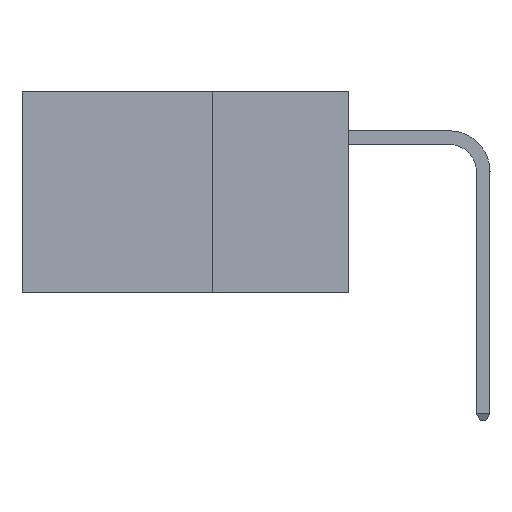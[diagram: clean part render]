
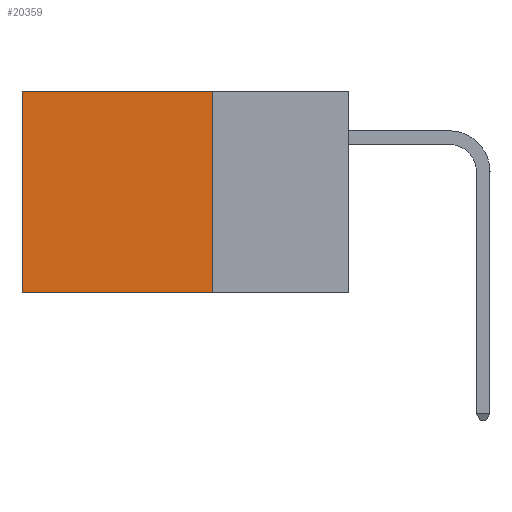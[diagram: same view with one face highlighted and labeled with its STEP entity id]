
A CAD part, left-side view. The second image highlights one B-rep face of the part: STEP entity #20359.
In plain terms, the highlighted planar face has unit normal (-1, 0, 0).
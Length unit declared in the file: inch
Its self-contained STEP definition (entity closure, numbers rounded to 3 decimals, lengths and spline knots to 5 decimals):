
#674 = VECTOR ( 'NONE', #28462, 39.37008 ) ;
#1531 = LINE ( 'NONE', #1655, #30522 ) ;
#1655 = CARTESIAN_POINT ( 'NONE',  ( 0.2875, 0.25, 0. ) ) ;
#2273 = DIRECTION ( 'NONE',  ( 0., 0., -1. ) ) ;
#3251 = CARTESIAN_POINT ( 'NONE',  ( 0.2875, 0.25, 0. ) ) ;
#4629 = VECTOR ( 'NONE', #25604, 39.37008 ) ;
#7291 = CARTESIAN_POINT ( 'NONE',  ( 0.2875, 0.25, -0.37 ) ) ;
#10611 = DIRECTION ( 'NONE',  ( 0., 1., 0. ) ) ;
#13455 = ORIENTED_EDGE ( 'NONE', *, *, #17270, .F. ) ;
#13987 = CARTESIAN_POINT ( 'NONE',  ( 0.2875, 0.25, -0.37 ) ) ;
#14924 = EDGE_CURVE ( 'NONE', #35983, #22302, #40123, .T. ) ;
#17270 = EDGE_CURVE ( 'NONE', #39607, #22302, #33731, .T. ) ;
#20359 = ADVANCED_FACE ( 'NONE', ( #41678 ), #40461, .F. ) ;
#22302 = VERTEX_POINT ( 'NONE', #36158 ) ;
#24394 = LINE ( 'NONE', #47756, #674 ) ;
#24557 = EDGE_LOOP ( 'NONE', ( #26845, #13455, #37991, #33889 ) ) ;
#25604 = DIRECTION ( 'NONE',  ( 0., 0., -1. ) ) ;
#26241 = EDGE_CURVE ( 'NONE', #45452, #35983, #1531, .T. ) ;
#26606 = VECTOR ( 'NONE', #10611, 39.37008 ) ;
#26845 = ORIENTED_EDGE ( 'NONE', *, *, #14924, .T. ) ;
#28206 = EDGE_CURVE ( 'NONE', #45452, #39607, #24394, .T. ) ;
#28462 = DIRECTION ( 'NONE',  ( 0., 0., -1. ) ) ;
#29075 = DIRECTION ( 'NONE',  ( 1., 0., 0. ) ) ;
#29636 = CARTESIAN_POINT ( 'NONE',  ( 0.2875, 0.6, 0. ) ) ;
#30522 = VECTOR ( 'NONE', #31423, 39.37008 ) ;
#31423 = DIRECTION ( 'NONE',  ( 0., 1., 0. ) ) ;
#33731 = LINE ( 'NONE', #7291, #26606 ) ;
#33889 = ORIENTED_EDGE ( 'NONE', *, *, #26241, .T. ) ;
#35983 = VERTEX_POINT ( 'NONE', #29636 ) ;
#36158 = CARTESIAN_POINT ( 'NONE',  ( 0.2875, 0.6, -0.37 ) ) ;
#37991 = ORIENTED_EDGE ( 'NONE', *, *, #28206, .F. ) ;
#39607 = VERTEX_POINT ( 'NONE', #13987 ) ;
#39979 = CARTESIAN_POINT ( 'NONE',  ( 0.2875, 0.25, 0. ) ) ;
#40123 = LINE ( 'NONE', #40622, #4629 ) ;
#40461 = PLANE ( 'NONE',  #46974 ) ;
#40622 = CARTESIAN_POINT ( 'NONE',  ( 0.2875, 0.6, 0. ) ) ;
#41678 = FACE_OUTER_BOUND ( 'NONE', #24557, .T. ) ;
#45452 = VERTEX_POINT ( 'NONE', #3251 ) ;
#46974 = AXIS2_PLACEMENT_3D ( 'NONE', #39979, #29075, #2273 ) ;
#47756 = CARTESIAN_POINT ( 'NONE',  ( 0.2875, 0.25, 0. ) ) ;
